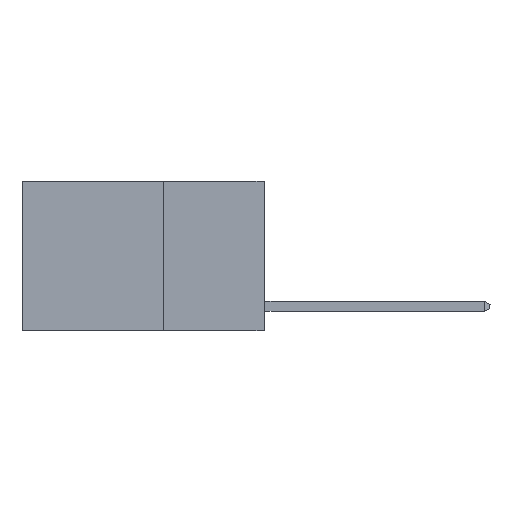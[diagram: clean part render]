
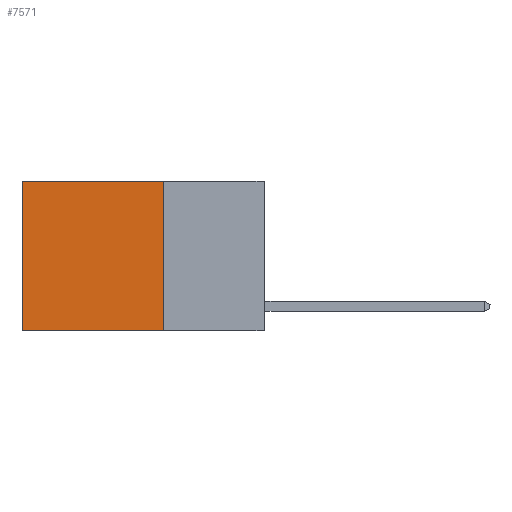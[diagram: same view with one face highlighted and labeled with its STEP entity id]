
A CAD part, left-side view. The second image highlights one B-rep face of the part: STEP entity #7571.
In plain terms, the highlighted planar face has unit normal (-1, 0, 0).
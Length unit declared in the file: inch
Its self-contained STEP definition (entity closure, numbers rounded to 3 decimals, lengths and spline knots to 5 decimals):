
#679 = LINE ( 'NONE', #13598, #19995 ) ;
#2311 = EDGE_CURVE ( 'NONE', #15361, #12905, #7868, .T. ) ;
#3804 = CARTESIAN_POINT ( 'NONE',  ( 0.2625, 0.25, 0. ) ) ;
#4540 = ORIENTED_EDGE ( 'NONE', *, *, #15698, .T. ) ;
#5569 = CARTESIAN_POINT ( 'NONE',  ( 0.2625, 0.25, 0. ) ) ;
#5944 = CARTESIAN_POINT ( 'NONE',  ( 0.2625, 0.25, 0. ) ) ;
#5971 = ORIENTED_EDGE ( 'NONE', *, *, #25867, .F. ) ;
#7571 = ADVANCED_FACE ( 'NONE', ( #12625 ), #27481, .F. ) ;
#7868 = LINE ( 'NONE', #25313, #14997 ) ;
#8028 = CARTESIAN_POINT ( 'NONE',  ( 0.2625, 0.25, 0. ) ) ;
#8478 = DIRECTION ( 'NONE',  ( 1., 0., 0. ) ) ;
#8721 = CARTESIAN_POINT ( 'NONE',  ( 0.2625, 0.6, 0. ) ) ;
#10476 = LINE ( 'NONE', #3804, #21022 ) ;
#10841 = ORIENTED_EDGE ( 'NONE', *, *, #20065, .T. ) ;
#11325 = DIRECTION ( 'NONE',  ( 0., 0., -1. ) ) ;
#11903 = VERTEX_POINT ( 'NONE', #5569 ) ;
#12215 = DIRECTION ( 'NONE',  ( 0., 0., -1. ) ) ;
#12625 = FACE_OUTER_BOUND ( 'NONE', #18635, .T. ) ;
#12905 = VERTEX_POINT ( 'NONE', #24164 ) ;
#13598 = CARTESIAN_POINT ( 'NONE',  ( 0.2625, 0.6, 0. ) ) ;
#14997 = VECTOR ( 'NONE', #22924, 39.37008 ) ;
#15361 = VERTEX_POINT ( 'NONE', #24399 ) ;
#15698 = EDGE_CURVE ( 'NONE', #21183, #12905, #679, .T. ) ;
#15805 = AXIS2_PLACEMENT_3D ( 'NONE', #5944, #8478, #12215 ) ;
#16717 = DIRECTION ( 'NONE',  ( 0., 1., 0. ) ) ;
#18635 = EDGE_LOOP ( 'NONE', ( #4540, #22311, #5971, #10841 ) ) ;
#19995 = VECTOR ( 'NONE', #11325, 39.37008 ) ;
#20065 = EDGE_CURVE ( 'NONE', #11903, #21183, #10476, .T. ) ;
#20806 = DIRECTION ( 'NONE',  ( 0., 0., -1. ) ) ;
#21022 = VECTOR ( 'NONE', #16717, 39.37008 ) ;
#21183 = VERTEX_POINT ( 'NONE', #8721 ) ;
#22311 = ORIENTED_EDGE ( 'NONE', *, *, #2311, .F. ) ;
#22924 = DIRECTION ( 'NONE',  ( 0., 1., 0. ) ) ;
#24164 = CARTESIAN_POINT ( 'NONE',  ( 0.2625, 0.6, -0.37 ) ) ;
#24399 = CARTESIAN_POINT ( 'NONE',  ( 0.2625, 0.25, -0.37 ) ) ;
#25313 = CARTESIAN_POINT ( 'NONE',  ( 0.2625, 0.25, -0.37 ) ) ;
#25867 = EDGE_CURVE ( 'NONE', #11903, #15361, #27736, .T. ) ;
#26489 = VECTOR ( 'NONE', #20806, 39.37008 ) ;
#27481 = PLANE ( 'NONE',  #15805 ) ;
#27736 = LINE ( 'NONE', #8028, #26489 ) ;
